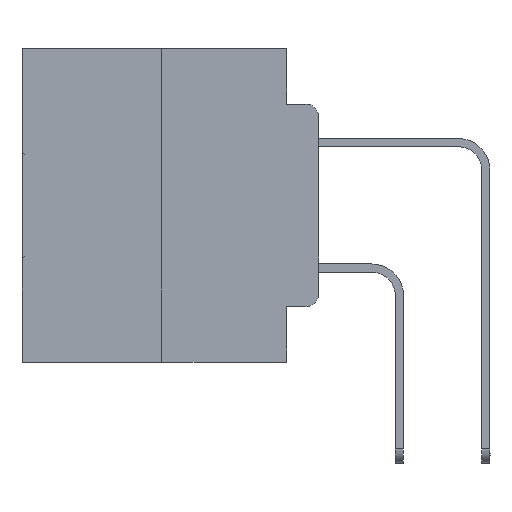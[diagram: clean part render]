
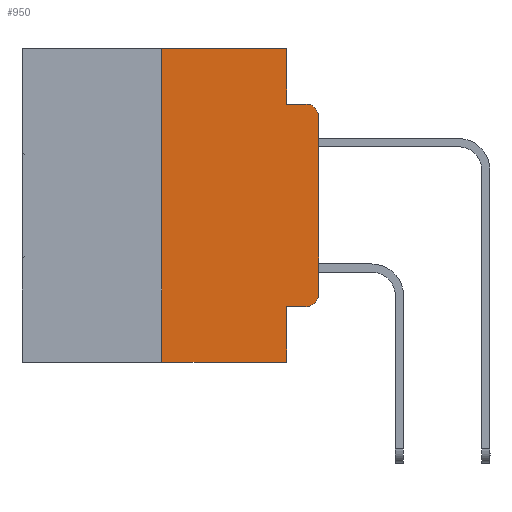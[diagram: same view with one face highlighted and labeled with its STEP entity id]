
A CAD part, left-side view. The second image highlights one B-rep face of the part: STEP entity #950.
In plain terms, the highlighted planar face has unit normal (-1, 0, 0).
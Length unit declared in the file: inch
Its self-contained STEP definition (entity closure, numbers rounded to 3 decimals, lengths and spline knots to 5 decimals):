
#333 = VERTEX_POINT ( 'NONE', #3399 ) ;
#893 = ORIENTED_EDGE ( 'NONE', *, *, #8472, .F. ) ;
#950 = ADVANCED_FACE ( 'NONE', ( #22112 ), #12472, .F. ) ;
#977 = DIRECTION ( 'NONE',  ( 0., 0., 1. ) ) ;
#1261 = DIRECTION ( 'NONE',  ( 0., 0., 1. ) ) ;
#1831 = CARTESIAN_POINT ( 'NONE',  ( 0., 0.25, 0. ) ) ;
#1850 = CARTESIAN_POINT ( 'NONE',  ( 0., 0.051, -0.4115 ) ) ;
#1992 = CARTESIAN_POINT ( 'NONE',  ( 0., 0.051, -0.5 ) ) ;
#2050 = CARTESIAN_POINT ( 'NONE',  ( 0., 0.051, -0.0885 ) ) ;
#2440 = LINE ( 'NONE', #4819, #7869 ) ;
#2705 = DIRECTION ( 'NONE',  ( 1., 0., 0. ) ) ;
#3097 = DIRECTION ( 'NONE',  ( -1., 0., 0. ) ) ;
#3399 = CARTESIAN_POINT ( 'NONE',  ( 0., 0., -0.1085 ) ) ;
#3684 = EDGE_CURVE ( 'NONE', #25445, #5250, #30028, .T. ) ;
#3828 = ORIENTED_EDGE ( 'NONE', *, *, #3684, .T. ) ;
#3870 = LINE ( 'NONE', #30329, #9462 ) ;
#4819 = CARTESIAN_POINT ( 'NONE',  ( 0., 0.473, -0.5 ) ) ;
#5250 = VERTEX_POINT ( 'NONE', #14574 ) ;
#5386 = CARTESIAN_POINT ( 'NONE',  ( 0., 0.02, -0.4115 ) ) ;
#6725 = VERTEX_POINT ( 'NONE', #7326 ) ;
#6933 = VECTOR ( 'NONE', #13068, 39.37008 ) ;
#7115 = VECTOR ( 'NONE', #26106, 39.37008 ) ;
#7326 = CARTESIAN_POINT ( 'NONE',  ( 0., 0.051, -0.4115 ) ) ;
#7869 = VECTOR ( 'NONE', #26558, 39.37008 ) ;
#7927 = CARTESIAN_POINT ( 'NONE',  ( 0., 0., 0. ) ) ;
#8322 = VECTOR ( 'NONE', #977, 39.37008 ) ;
#8419 = CARTESIAN_POINT ( 'NONE',  ( 0., 0.051, -0.0885 ) ) ;
#8472 = EDGE_CURVE ( 'NONE', #12416, #16760, #16460, .T. ) ;
#8658 = CARTESIAN_POINT ( 'NONE',  ( 0., 0.25, -0.5 ) ) ;
#8914 = CARTESIAN_POINT ( 'NONE',  ( 0., 0.02, -0.1085 ) ) ;
#9263 = EDGE_CURVE ( 'NONE', #333, #15486, #12127, .T. ) ;
#9424 = EDGE_CURVE ( 'NONE', #16760, #25723, #26256, .T. ) ;
#9462 = VECTOR ( 'NONE', #30486, 39.37008 ) ;
#9705 = VECTOR ( 'NONE', #1261, 39.37008 ) ;
#10780 = LINE ( 'NONE', #8419, #24202 ) ;
#10919 = CARTESIAN_POINT ( 'NONE',  ( 0., 0.02, -0.3915 ) ) ;
#11095 = DIRECTION ( 'NONE',  ( 0., -1., 0. ) ) ;
#12127 = CIRCLE ( 'NONE', #29728, 0.02 ) ;
#12416 = VERTEX_POINT ( 'NONE', #1831 ) ;
#12472 = PLANE ( 'NONE',  #30778 ) ;
#13068 = DIRECTION ( 'NONE',  ( 0., -1., 0. ) ) ;
#13770 = DIRECTION ( 'NONE',  ( 0., -1., 0. ) ) ;
#13940 = ORIENTED_EDGE ( 'NONE', *, *, #9424, .F. ) ;
#14281 = DIRECTION ( 'NONE',  ( -1., 0., 0. ) ) ;
#14381 = CARTESIAN_POINT ( 'NONE',  ( 0., 0.02, -0.0885 ) ) ;
#14574 = CARTESIAN_POINT ( 'NONE',  ( 0., 0., -0.3915 ) ) ;
#15197 = LINE ( 'NONE', #7927, #8322 ) ;
#15469 = CARTESIAN_POINT ( 'NONE',  ( 0., 0.25, 0. ) ) ;
#15486 = VERTEX_POINT ( 'NONE', #14381 ) ;
#16460 = LINE ( 'NONE', #26074, #19647 ) ;
#16497 = CARTESIAN_POINT ( 'NONE',  ( 0., 0.051, 0. ) ) ;
#16760 = VERTEX_POINT ( 'NONE', #19264 ) ;
#16942 = EDGE_CURVE ( 'NONE', #24319, #12416, #27135, .T. ) ;
#17994 = LINE ( 'NONE', #1850, #6933 ) ;
#19264 = CARTESIAN_POINT ( 'NONE',  ( 0., 0.051, 0. ) ) ;
#19266 = EDGE_CURVE ( 'NONE', #5250, #333, #15197, .T. ) ;
#19423 = DIRECTION ( 'NONE',  ( 0., 0., -1. ) ) ;
#19647 = VECTOR ( 'NONE', #13770, 39.37008 ) ;
#21719 = EDGE_CURVE ( 'NONE', #24319, #27986, #2440, .T. ) ;
#21751 = ORIENTED_EDGE ( 'NONE', *, *, #23633, .F. ) ;
#22112 = FACE_OUTER_BOUND ( 'NONE', #23315, .T. ) ;
#22213 = ORIENTED_EDGE ( 'NONE', *, *, #16942, .F. ) ;
#23153 = EDGE_CURVE ( 'NONE', #6725, #25445, #17994, .T. ) ;
#23315 = EDGE_LOOP ( 'NONE', ( #24787, #26975, #28559, #13940, #893, #22213, #30094, #21751, #23496, #3828 ) ) ;
#23496 = ORIENTED_EDGE ( 'NONE', *, *, #23153, .T. ) ;
#23633 = EDGE_CURVE ( 'NONE', #6725, #27986, #3870, .T. ) ;
#23904 = DIRECTION ( 'NONE',  ( 0., 0., -1. ) ) ;
#24202 = VECTOR ( 'NONE', #11095, 39.37008 ) ;
#24319 = VERTEX_POINT ( 'NONE', #8658 ) ;
#24787 = ORIENTED_EDGE ( 'NONE', *, *, #19266, .T. ) ;
#25445 = VERTEX_POINT ( 'NONE', #5386 ) ;
#25723 = VERTEX_POINT ( 'NONE', #2050 ) ;
#26074 = CARTESIAN_POINT ( 'NONE',  ( 0., 0.473, 0. ) ) ;
#26106 = DIRECTION ( 'NONE',  ( 0., 0., -1. ) ) ;
#26256 = LINE ( 'NONE', #16497, #7115 ) ;
#26513 = CARTESIAN_POINT ( 'NONE',  ( 0., 0.473, 0. ) ) ;
#26537 = EDGE_CURVE ( 'NONE', #25723, #15486, #10780, .T. ) ;
#26558 = DIRECTION ( 'NONE',  ( 0., -1., 0. ) ) ;
#26975 = ORIENTED_EDGE ( 'NONE', *, *, #9263, .T. ) ;
#27135 = LINE ( 'NONE', #15469, #9705 ) ;
#27986 = VERTEX_POINT ( 'NONE', #1992 ) ;
#28559 = ORIENTED_EDGE ( 'NONE', *, *, #26537, .F. ) ;
#29526 = AXIS2_PLACEMENT_3D ( 'NONE', #10919, #3097, #30148 ) ;
#29728 = AXIS2_PLACEMENT_3D ( 'NONE', #8914, #14281, #23904 ) ;
#30028 = CIRCLE ( 'NONE', #29526, 0.02 ) ;
#30094 = ORIENTED_EDGE ( 'NONE', *, *, #21719, .T. ) ;
#30148 = DIRECTION ( 'NONE',  ( 0., 0., -1. ) ) ;
#30329 = CARTESIAN_POINT ( 'NONE',  ( 0., 0.051, 0. ) ) ;
#30486 = DIRECTION ( 'NONE',  ( 0., 0., -1. ) ) ;
#30778 = AXIS2_PLACEMENT_3D ( 'NONE', #26513, #2705, #19423 ) ;
